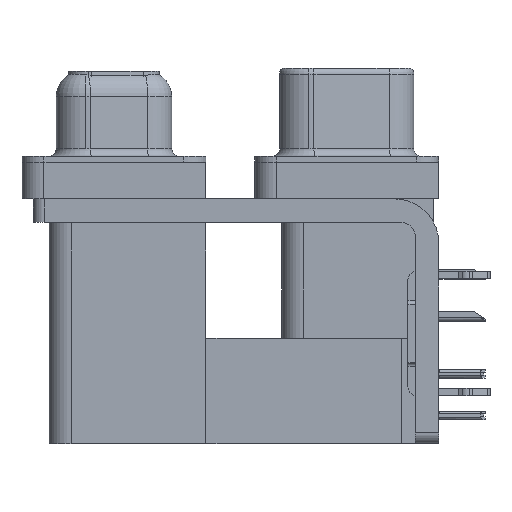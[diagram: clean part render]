
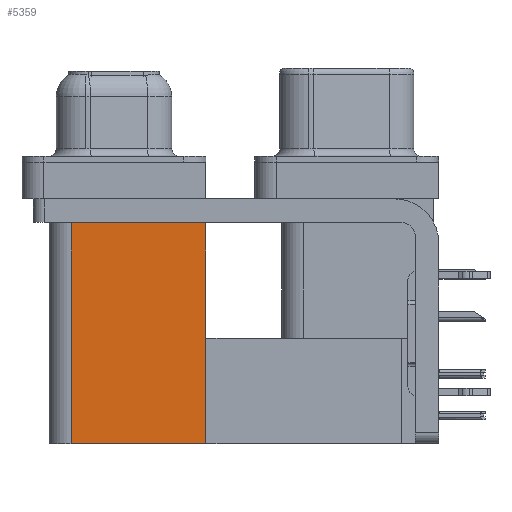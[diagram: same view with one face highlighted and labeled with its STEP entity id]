
A CAD part, left-side view. The second image highlights one B-rep face of the part: STEP entity #5359.
In plain terms, the highlighted planar face has unit normal (-1, 0, 0).
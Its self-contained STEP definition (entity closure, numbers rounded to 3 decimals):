
#7 = VERTEX_POINT ( 'NONE', #6459 ) ;
#5305 = PLANE ( 'NONE',  #11402 ) ;
#5359 = ADVANCED_FACE ( 'NONE', ( #20362 ), #5305, .F. ) ;
#6459 = CARTESIAN_POINT ( 'NONE',  ( 3.765, 9.6, -2.5 ) ) ;
#6718 = CARTESIAN_POINT ( 'NONE',  ( 3.765, 18.8, -2.5 ) ) ;
#6960 = EDGE_CURVE ( 'NONE', #7, #18532, #38289, .T. ) ;
#11402 = AXIS2_PLACEMENT_3D ( 'NONE', #20132, #16372, #12611 ) ;
#11682 = DIRECTION ( 'NONE',  ( 0., 0., 1. ) ) ;
#12565 = DIRECTION ( 'NONE',  ( 0., 1., 0. ) ) ;
#12611 = DIRECTION ( 'NONE',  ( 0., 0., -1. ) ) ;
#12636 = EDGE_CURVE ( 'NONE', #14296, #18532, #16398, .T. ) ;
#14255 = VECTOR ( 'NONE', #34596, 1000. ) ;
#14296 = VERTEX_POINT ( 'NONE', #46313 ) ;
#16372 = DIRECTION ( 'NONE',  ( 1., 0., 0. ) ) ;
#16398 = LINE ( 'NONE', #45874, #14255 ) ;
#18064 = ORIENTED_EDGE ( 'NONE', *, *, #42889, .F. ) ;
#18532 = VERTEX_POINT ( 'NONE', #6718 ) ;
#20132 = CARTESIAN_POINT ( 'NONE',  ( 3.765, 9.6, -19.2 ) ) ;
#20362 = FACE_OUTER_BOUND ( 'NONE', #35807, .T. ) ;
#25852 = LINE ( 'NONE', #36247, #29872 ) ;
#26763 = CARTESIAN_POINT ( 'NONE',  ( 3.765, 9.6, -2.5 ) ) ;
#26941 = CARTESIAN_POINT ( 'NONE',  ( 3.765, 9.6, -19.2 ) ) ;
#27303 = CARTESIAN_POINT ( 'NONE',  ( 3.765, 9.6, -19.2 ) ) ;
#29395 = VECTOR ( 'NONE', #41696, 1000. ) ;
#29510 = ORIENTED_EDGE ( 'NONE', *, *, #12636, .F. ) ;
#29872 = VECTOR ( 'NONE', #11682, 1000. ) ;
#31274 = ORIENTED_EDGE ( 'NONE', *, *, #6960, .T. ) ;
#32459 = EDGE_CURVE ( 'NONE', #33057, #7, #25852, .T. ) ;
#33057 = VERTEX_POINT ( 'NONE', #26941 ) ;
#34596 = DIRECTION ( 'NONE',  ( 0., 0., 1. ) ) ;
#35471 = VECTOR ( 'NONE', #12565, 1000. ) ;
#35807 = EDGE_LOOP ( 'NONE', ( #31274, #29510, #18064, #37087 ) ) ;
#36247 = CARTESIAN_POINT ( 'NONE',  ( 3.765, 9.6, -19.2 ) ) ;
#37087 = ORIENTED_EDGE ( 'NONE', *, *, #32459, .T. ) ;
#37932 = LINE ( 'NONE', #27303, #29395 ) ;
#38289 = LINE ( 'NONE', #26763, #35471 ) ;
#41696 = DIRECTION ( 'NONE',  ( 0., 1., 0. ) ) ;
#42889 = EDGE_CURVE ( 'NONE', #33057, #14296, #37932, .T. ) ;
#45874 = CARTESIAN_POINT ( 'NONE',  ( 3.765, 18.8, -19.2 ) ) ;
#46313 = CARTESIAN_POINT ( 'NONE',  ( 3.765, 18.8, -19.2 ) ) ;
